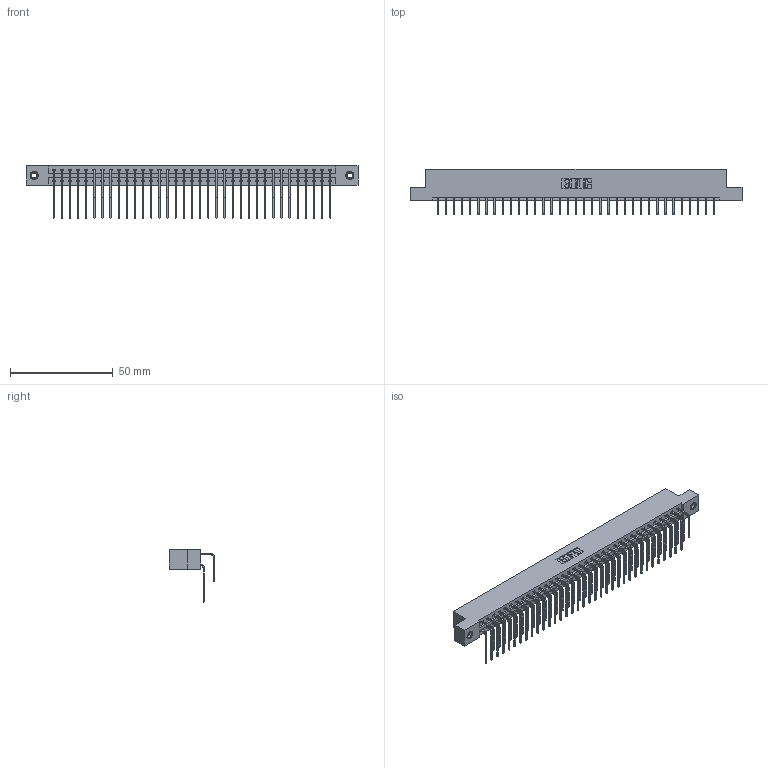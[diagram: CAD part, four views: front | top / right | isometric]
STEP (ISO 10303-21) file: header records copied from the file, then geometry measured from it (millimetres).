
FILE_DESCRIPTION (( 'STEP AP203' ), '1' );
FILE_NAME ('337-070-558-207.STEP', '2019-10-10T01:49:22', ( '' ), ( '' ), 'SwSTEP 2.0', 'SolidWorks 2016', '' );
FILE_SCHEMA (( 'CONFIG_CONTROL_DESIGN' ));
Length unit declared in the file: inch
Products named in the file (5): 345-292-001_558 Tail - 2; 345-250-001_345-250-005-103; 337-070-558-207; 337 Part_Flush Mounting Lugs - 0.156 Dia-TI; 345-292-001_558 559 Tail - 1
Assembly tree (73 placements, depth 2):
  337-070-558-207
    337 Part_Flush Mounting Lugs - 0.156 Dia-TI
    345-292-001_558 559 Tail - 1  x35
    345-292-001_558 Tail - 2  x35
    345-250-001_345-250-005-103  x2
Bounding box: 161.7 x 22.17 x 25.53 mm (x, y, z)
Volume: 17338 mm3; surface area: 21596.2 mm2
Topology: 73 solids, 73 shells, 4094 faces, 12137 edges, 7990 vertices
Faces by surface type: plane 2902, cylinder 1176, cone 12, torus 4
Entity records: 31012 total; most frequent: CARTESIAN_POINT 5256, ORIENTED_EDGE 5134, DIRECTION 4497, EDGE_CURVE 2567, VECTOR 2379, LINE 2379, VERTEX_POINT 1704, AXIS2_PLACEMENT_3D 1059
